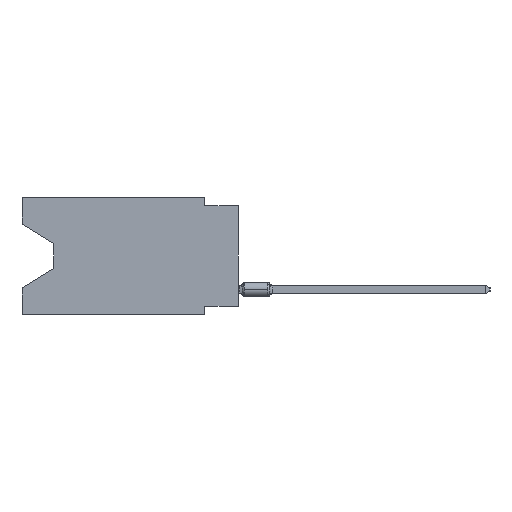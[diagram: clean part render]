
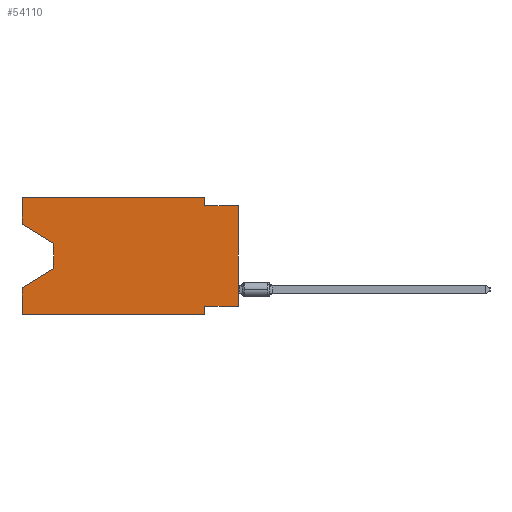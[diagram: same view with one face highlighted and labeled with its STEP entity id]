
A CAD part, left-side view. The second image highlights one B-rep face of the part: STEP entity #54110.
In plain terms, the highlighted planar face has unit normal (-1, 0, 0).
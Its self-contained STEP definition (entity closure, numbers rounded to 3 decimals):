
#90 = FACE_OUTER_BOUND ( 'NONE', #20131, .T. ) ;
#394 = DIRECTION ( 'NONE',  ( 1., 0., 0. ) ) ;
#431 = CARTESIAN_POINT ( 'NONE',  ( 0., 16.383, -8.89 ) ) ;
#660 = LINE ( 'NONE', #39740, #52497 ) ;
#2408 = LINE ( 'NONE', #40861, #38466 ) ;
#2441 = VECTOR ( 'NONE', #14485, 1000. ) ;
#3134 = LINE ( 'NONE', #37698, #7698 ) ;
#3806 = DIRECTION ( 'NONE',  ( 0., 1., 0. ) ) ;
#4010 = LINE ( 'NONE', #23546, #4314 ) ;
#4223 = CARTESIAN_POINT ( 'NONE',  ( 0., 16.383, -6.852 ) ) ;
#4314 = VECTOR ( 'NONE', #51766, 1000. ) ;
#6240 = CARTESIAN_POINT ( 'NONE',  ( 0., 13.97, -3.505 ) ) ;
#7222 = ORIENTED_EDGE ( 'NONE', *, *, #50952, .T. ) ;
#7698 = VECTOR ( 'NONE', #27777, 1000. ) ;
#8307 = LINE ( 'NONE', #56027, #22091 ) ;
#8927 = CARTESIAN_POINT ( 'NONE',  ( 0., 0., -8.255 ) ) ;
#9095 = VECTOR ( 'NONE', #57898, 1000. ) ;
#9648 = ORIENTED_EDGE ( 'NONE', *, *, #42901, .T. ) ;
#10202 = ORIENTED_EDGE ( 'NONE', *, *, #13460, .F. ) ;
#10995 = DIRECTION ( 'NONE',  ( 0., -0.855, -0.519 ) ) ;
#11327 = VECTOR ( 'NONE', #35219, 1000. ) ;
#11372 = EDGE_CURVE ( 'NONE', #11905, #61796, #4010, .T. ) ;
#11905 = VERTEX_POINT ( 'NONE', #63157 ) ;
#13303 = AXIS2_PLACEMENT_3D ( 'NONE', #49713, #394, #18993 ) ;
#13392 = LINE ( 'NONE', #52788, #9095 ) ;
#13460 = EDGE_CURVE ( 'NONE', #61796, #33710, #38525, .T. ) ;
#14485 = DIRECTION ( 'NONE',  ( 0., 0., -1. ) ) ;
#14605 = CARTESIAN_POINT ( 'NONE',  ( 0., 16.383, -2.038 ) ) ;
#15559 = ORIENTED_EDGE ( 'NONE', *, *, #54792, .T. ) ;
#15700 = VERTEX_POINT ( 'NONE', #29834 ) ;
#16054 = ORIENTED_EDGE ( 'NONE', *, *, #44698, .F. ) ;
#17756 = VECTOR ( 'NONE', #10995, 1000. ) ;
#17948 = CARTESIAN_POINT ( 'NONE',  ( 0., 13.97, -3.505 ) ) ;
#18665 = CARTESIAN_POINT ( 'NONE',  ( 0., 2.54, 0. ) ) ;
#18993 = DIRECTION ( 'NONE',  ( 0., 0., -1. ) ) ;
#19009 = CARTESIAN_POINT ( 'NONE',  ( 0., 2.54, -8.89 ) ) ;
#19170 = LINE ( 'NONE', #8927, #57647 ) ;
#19628 = PLANE ( 'NONE',  #13303 ) ;
#20131 = EDGE_LOOP ( 'NONE', ( #25444, #7222, #15559, #31785, #9648, #49494, #57779, #58494, #41935, #10202, #48816, #16054 ) ) ;
#20160 = VERTEX_POINT ( 'NONE', #17948 ) ;
#20803 = CARTESIAN_POINT ( 'NONE',  ( 0., 2.54, -8.89 ) ) ;
#22091 = VECTOR ( 'NONE', #36811, 1000. ) ;
#23546 = CARTESIAN_POINT ( 'NONE',  ( 0., 16.383, 0. ) ) ;
#23577 = CARTESIAN_POINT ( 'NONE',  ( 0., 0., -8.255 ) ) ;
#25407 = VERTEX_POINT ( 'NONE', #54326 ) ;
#25444 = ORIENTED_EDGE ( 'NONE', *, *, #39739, .T. ) ;
#26550 = LINE ( 'NONE', #20803, #11327 ) ;
#27777 = DIRECTION ( 'NONE',  ( 0., 0., 1. ) ) ;
#29597 = LINE ( 'NONE', #6240, #59681 ) ;
#29834 = CARTESIAN_POINT ( 'NONE',  ( 0., 0., -0.635 ) ) ;
#30110 = VERTEX_POINT ( 'NONE', #4223 ) ;
#30770 = EDGE_CURVE ( 'NONE', #41108, #30110, #3134, .T. ) ;
#31236 = DIRECTION ( 'NONE',  ( 0., -1., 0. ) ) ;
#31381 = VECTOR ( 'NONE', #48539, 1000. ) ;
#31785 = ORIENTED_EDGE ( 'NONE', *, *, #30770, .F. ) ;
#32481 = VERTEX_POINT ( 'NONE', #14605 ) ;
#32545 = LINE ( 'NONE', #57194, #31381 ) ;
#33710 = VERTEX_POINT ( 'NONE', #39598 ) ;
#35219 = DIRECTION ( 'NONE',  ( 0., 0., -1. ) ) ;
#36811 = DIRECTION ( 'NONE',  ( 0., -1., 0. ) ) ;
#37698 = CARTESIAN_POINT ( 'NONE',  ( 0., 16.383, 0. ) ) ;
#37975 = VERTEX_POINT ( 'NONE', #39099 ) ;
#38466 = VECTOR ( 'NONE', #31236, 1000. ) ;
#38525 = LINE ( 'NONE', #18665, #2441 ) ;
#39099 = CARTESIAN_POINT ( 'NONE',  ( 0., 2.54, -8.255 ) ) ;
#39471 = EDGE_CURVE ( 'NONE', #62094, #15700, #660, .T. ) ;
#39598 = CARTESIAN_POINT ( 'NONE',  ( 0., 2.54, -0.635 ) ) ;
#39739 = EDGE_CURVE ( 'NONE', #32481, #20160, #44928, .T. ) ;
#39740 = CARTESIAN_POINT ( 'NONE',  ( 0., 0., 0. ) ) ;
#40112 = EDGE_CURVE ( 'NONE', #62094, #37975, #19170, .T. ) ;
#40281 = CARTESIAN_POINT ( 'NONE',  ( 0., 2.54, 0. ) ) ;
#40861 = CARTESIAN_POINT ( 'NONE',  ( 0., 0., -0.635 ) ) ;
#41108 = VERTEX_POINT ( 'NONE', #431 ) ;
#41935 = ORIENTED_EDGE ( 'NONE', *, *, #43160, .F. ) ;
#42901 = EDGE_CURVE ( 'NONE', #41108, #45459, #8307, .T. ) ;
#43160 = EDGE_CURVE ( 'NONE', #33710, #15700, #2408, .T. ) ;
#44653 = DIRECTION ( 'NONE',  ( 0., 0., -1. ) ) ;
#44698 = EDGE_CURVE ( 'NONE', #32481, #11905, #13392, .T. ) ;
#44928 = LINE ( 'NONE', #45575, #17756 ) ;
#45459 = VERTEX_POINT ( 'NONE', #19009 ) ;
#45575 = CARTESIAN_POINT ( 'NONE',  ( 0., 16.383, -2.038 ) ) ;
#48539 = DIRECTION ( 'NONE',  ( 0., 0.855, -0.519 ) ) ;
#48816 = ORIENTED_EDGE ( 'NONE', *, *, #11372, .F. ) ;
#49494 = ORIENTED_EDGE ( 'NONE', *, *, #60216, .F. ) ;
#49713 = CARTESIAN_POINT ( 'NONE',  ( 0., 16.383, 0. ) ) ;
#50952 = EDGE_CURVE ( 'NONE', #20160, #25407, #29597, .T. ) ;
#51766 = DIRECTION ( 'NONE',  ( 0., -1., 0. ) ) ;
#52497 = VECTOR ( 'NONE', #61151, 1000. ) ;
#52788 = CARTESIAN_POINT ( 'NONE',  ( 0., 16.383, 0. ) ) ;
#54110 = ADVANCED_FACE ( 'NONE', ( #90 ), #19628, .F. ) ;
#54326 = CARTESIAN_POINT ( 'NONE',  ( 0., 13.97, -5.385 ) ) ;
#54792 = EDGE_CURVE ( 'NONE', #25407, #30110, #32545, .T. ) ;
#56027 = CARTESIAN_POINT ( 'NONE',  ( 0., 16.383, -8.89 ) ) ;
#57194 = CARTESIAN_POINT ( 'NONE',  ( 0., 13.97, -5.385 ) ) ;
#57647 = VECTOR ( 'NONE', #3806, 1000. ) ;
#57779 = ORIENTED_EDGE ( 'NONE', *, *, #40112, .F. ) ;
#57898 = DIRECTION ( 'NONE',  ( 0., 0., 1. ) ) ;
#58494 = ORIENTED_EDGE ( 'NONE', *, *, #39471, .T. ) ;
#59681 = VECTOR ( 'NONE', #44653, 1000. ) ;
#60216 = EDGE_CURVE ( 'NONE', #37975, #45459, #26550, .T. ) ;
#61151 = DIRECTION ( 'NONE',  ( 0., 0., 1. ) ) ;
#61796 = VERTEX_POINT ( 'NONE', #40281 ) ;
#62094 = VERTEX_POINT ( 'NONE', #23577 ) ;
#63157 = CARTESIAN_POINT ( 'NONE',  ( 0., 16.383, 0. ) ) ;
